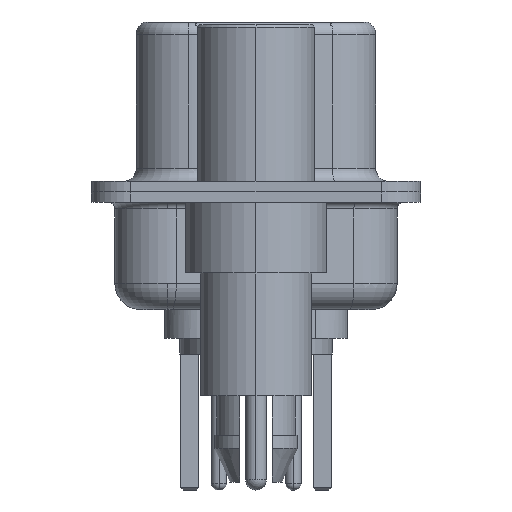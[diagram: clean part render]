
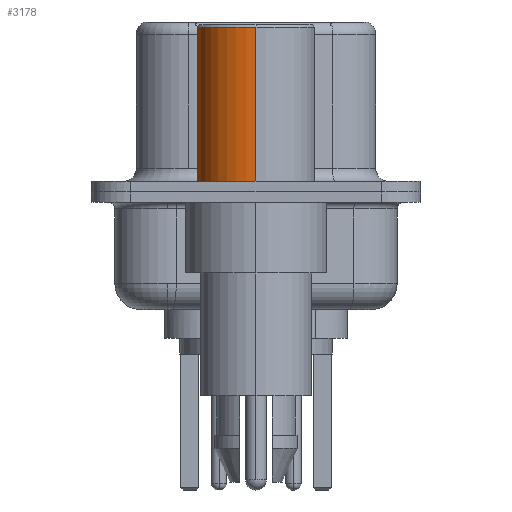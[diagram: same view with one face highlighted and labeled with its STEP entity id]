
A CAD part, left-side view. The second image highlights one B-rep face of the part: STEP entity #3178.
In plain terms, the highlighted cylindrical face has radius 2.25 mm (diameter 4.5 mm), a partial arc.
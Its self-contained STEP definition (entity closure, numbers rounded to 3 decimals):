
#91 = CARTESIAN_POINT ( 'NONE',  ( 0., 0., 6.3 ) ) ;
#106 = CYLINDRICAL_SURFACE ( 'NONE', #3510, 2.25 ) ;
#2046 = DIRECTION ( 'NONE',  ( 1., 0., 0. ) ) ;
#2133 = CARTESIAN_POINT ( 'NONE',  ( -2.25, 0., 0.581 ) ) ;
#2991 = AXIS2_PLACEMENT_3D ( 'NONE', #21890, #10012, #23855 ) ;
#3014 = LINE ( 'NONE', #8410, #18217 ) ;
#3178 = ADVANCED_FACE ( 'NONE', ( #10606 ), #106, .T. ) ;
#3510 = AXIS2_PLACEMENT_3D ( 'NONE', #14349, #10596, #10679 ) ;
#4953 = ORIENTED_EDGE ( 'NONE', *, *, #15663, .F. ) ;
#5324 = VERTEX_POINT ( 'NONE', #12959 ) ;
#7150 = EDGE_CURVE ( 'NONE', #5324, #19320, #12047, .T. ) ;
#8410 = CARTESIAN_POINT ( 'NONE',  ( 2.25, 0., 0.581 ) ) ;
#10012 = DIRECTION ( 'NONE',  ( 0., 0., 1. ) ) ;
#10413 = DIRECTION ( 'NONE',  ( 0., 0., 1. ) ) ;
#10596 = DIRECTION ( 'NONE',  ( 0., 0., 1. ) ) ;
#10606 = FACE_OUTER_BOUND ( 'NONE', #18160, .T. ) ;
#10679 = DIRECTION ( 'NONE',  ( 1., 0., 0. ) ) ;
#11261 = ORIENTED_EDGE ( 'NONE', *, *, #7150, .T. ) ;
#12047 = LINE ( 'NONE', #2133, #21316 ) ;
#12127 = CIRCLE ( 'NONE', #2991, 2.25 ) ;
#12631 = CIRCLE ( 'NONE', #21704, 2.25 ) ;
#12959 = CARTESIAN_POINT ( 'NONE',  ( -2.25, 0., 0.4 ) ) ;
#13946 = DIRECTION ( 'NONE',  ( 0., 0., 1. ) ) ;
#14349 = CARTESIAN_POINT ( 'NONE',  ( 0., 0., 0.581 ) ) ;
#15663 = EDGE_CURVE ( 'NONE', #19194, #20550, #3014, .T. ) ;
#16182 = DIRECTION ( 'NONE',  ( 0., 0., 1. ) ) ;
#16321 = CARTESIAN_POINT ( 'NONE',  ( 2.25, 0., 0.4 ) ) ;
#16847 = EDGE_CURVE ( 'NONE', #20550, #19320, #12631, .T. ) ;
#17288 = CARTESIAN_POINT ( 'NONE',  ( 2.25, 0., 6.3 ) ) ;
#18160 = EDGE_LOOP ( 'NONE', ( #20973, #11261, #24534, #4953 ) ) ;
#18217 = VECTOR ( 'NONE', #10413, 1000. ) ;
#19194 = VERTEX_POINT ( 'NONE', #16321 ) ;
#19320 = VERTEX_POINT ( 'NONE', #20629 ) ;
#20550 = VERTEX_POINT ( 'NONE', #17288 ) ;
#20629 = CARTESIAN_POINT ( 'NONE',  ( -2.25, 0., 6.3 ) ) ;
#20973 = ORIENTED_EDGE ( 'NONE', *, *, #21815, .T. ) ;
#21316 = VECTOR ( 'NONE', #16182, 1000. ) ;
#21704 = AXIS2_PLACEMENT_3D ( 'NONE', #91, #13946, #2046 ) ;
#21815 = EDGE_CURVE ( 'NONE', #19194, #5324, #12127, .T. ) ;
#21890 = CARTESIAN_POINT ( 'NONE',  ( 0., 0., 0.4 ) ) ;
#23855 = DIRECTION ( 'NONE',  ( 1., 0., 0. ) ) ;
#24534 = ORIENTED_EDGE ( 'NONE', *, *, #16847, .F. ) ;
